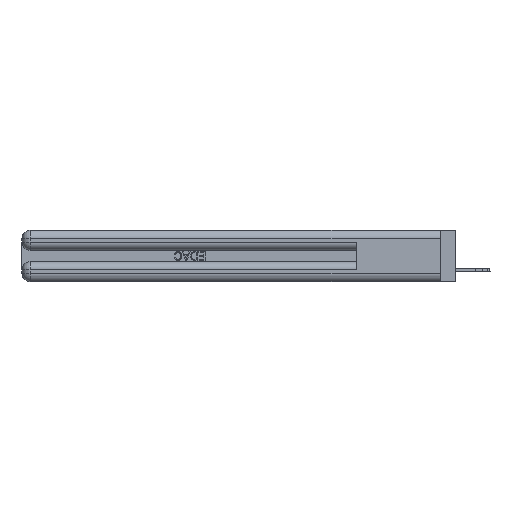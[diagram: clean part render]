
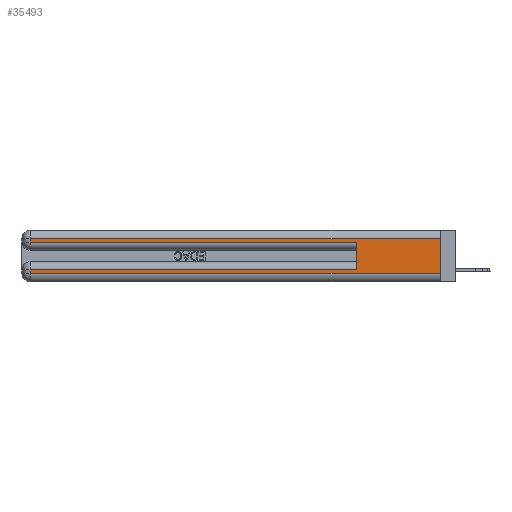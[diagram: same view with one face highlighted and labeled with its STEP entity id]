
A CAD part, left-side view. The second image highlights one B-rep face of the part: STEP entity #35493.
In plain terms, the highlighted planar face has unit normal (-1, 0, 0).
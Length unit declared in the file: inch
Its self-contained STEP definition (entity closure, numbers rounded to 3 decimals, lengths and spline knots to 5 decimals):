
#1325 = ORIENTED_EDGE ( 'NONE', *, *, #3280, .T. ) ;
#1948 = PLANE ( 'NONE',  #37656 ) ;
#2140 = DIRECTION ( 'NONE',  ( 0., 0., -1. ) ) ;
#2930 = VERTEX_POINT ( 'NONE', #23353 ) ;
#3280 = EDGE_CURVE ( 'NONE', #31481, #2930, #23337, .T. ) ;
#3364 = CARTESIAN_POINT ( 'NONE',  ( 0., 0., 0.31 ) ) ;
#3523 = VECTOR ( 'NONE', #14774, 39.37008 ) ;
#3614 = EDGE_CURVE ( 'NONE', #2930, #20798, #17515, .T. ) ;
#4989 = VECTOR ( 'NONE', #32613, 39.37008 ) ;
#5030 = CARTESIAN_POINT ( 'NONE',  ( 0., 0., 0.06 ) ) ;
#5789 = LINE ( 'NONE', #5030, #34237 ) ;
#6220 = LINE ( 'NONE', #10627, #21647 ) ;
#8026 = DIRECTION ( 'NONE',  ( 1., 0., 0. ) ) ;
#8174 = VECTOR ( 'NONE', #14922, 39.37008 ) ;
#8449 = ORIENTED_EDGE ( 'NONE', *, *, #36669, .T. ) ;
#8536 = VERTEX_POINT ( 'NONE', #16833 ) ;
#10357 = CARTESIAN_POINT ( 'NONE',  ( 0., 0., 0.31 ) ) ;
#10627 = CARTESIAN_POINT ( 'NONE',  ( 0., 0., 0.085 ) ) ;
#11812 = CARTESIAN_POINT ( 'NONE',  ( 0., 0.6, 0.145 ) ) ;
#11823 = CARTESIAN_POINT ( 'NONE',  ( 0., 2.94, 0.06 ) ) ;
#13100 = CARTESIAN_POINT ( 'NONE',  ( 0., 0., 0.37 ) ) ;
#13444 = VERTEX_POINT ( 'NONE', #30317 ) ;
#13823 = LINE ( 'NONE', #17106, #23493 ) ;
#13838 = VECTOR ( 'NONE', #22507, 39.37008 ) ;
#14729 = EDGE_CURVE ( 'NONE', #14881, #20798, #38062, .T. ) ;
#14774 = DIRECTION ( 'NONE',  ( 0., 0., -1. ) ) ;
#14881 = VERTEX_POINT ( 'NONE', #22222 ) ;
#14922 = DIRECTION ( 'NONE',  ( 0., 0., 1. ) ) ;
#14942 = ORIENTED_EDGE ( 'NONE', *, *, #26056, .T. ) ;
#15042 = EDGE_LOOP ( 'NONE', ( #24787, #33107, #1325, #31427, #30778, #14942, #8449, #38339 ) ) ;
#16712 = DIRECTION ( 'NONE',  ( 0., -1., 0. ) ) ;
#16833 = CARTESIAN_POINT ( 'NONE',  ( 0., 0., 0.06 ) ) ;
#17106 = CARTESIAN_POINT ( 'NONE',  ( 0., 2.94, 0.37 ) ) ;
#17515 = LINE ( 'NONE', #38099, #4989 ) ;
#18648 = VECTOR ( 'NONE', #34614, 39.37008 ) ;
#20024 = DIRECTION ( 'NONE',  ( 0., 0., -1. ) ) ;
#20262 = FACE_OUTER_BOUND ( 'NONE', #15042, .T. ) ;
#20798 = VERTEX_POINT ( 'NONE', #31462 ) ;
#21647 = VECTOR ( 'NONE', #35519, 39.37008 ) ;
#22222 = CARTESIAN_POINT ( 'NONE',  ( 0., 0.6, 0.085 ) ) ;
#22507 = DIRECTION ( 'NONE',  ( 0., 1., 0. ) ) ;
#23337 = LINE ( 'NONE', #33353, #3523 ) ;
#23353 = CARTESIAN_POINT ( 'NONE',  ( 0., 2.94, 0.285 ) ) ;
#23493 = VECTOR ( 'NONE', #2140, 39.37008 ) ;
#24787 = ORIENTED_EDGE ( 'NONE', *, *, #36968, .F. ) ;
#25267 = EDGE_CURVE ( 'NONE', #29333, #8536, #5789, .T. ) ;
#26056 = EDGE_CURVE ( 'NONE', #14881, #13444, #6220, .T. ) ;
#29333 = VERTEX_POINT ( 'NONE', #11823 ) ;
#30243 = EDGE_CURVE ( 'NONE', #30724, #31481, #36104, .T. ) ;
#30317 = CARTESIAN_POINT ( 'NONE',  ( 0., 2.94, 0.085 ) ) ;
#30724 = VERTEX_POINT ( 'NONE', #3364 ) ;
#30778 = ORIENTED_EDGE ( 'NONE', *, *, #14729, .F. ) ;
#31427 = ORIENTED_EDGE ( 'NONE', *, *, #3614, .T. ) ;
#31462 = CARTESIAN_POINT ( 'NONE',  ( 0., 0.6, 0.285 ) ) ;
#31481 = VERTEX_POINT ( 'NONE', #34067 ) ;
#32613 = DIRECTION ( 'NONE',  ( 0., -1., 0. ) ) ;
#33107 = ORIENTED_EDGE ( 'NONE', *, *, #30243, .T. ) ;
#33264 = LINE ( 'NONE', #13100, #18648 ) ;
#33353 = CARTESIAN_POINT ( 'NONE',  ( 0., 2.94, 0.37 ) ) ;
#34067 = CARTESIAN_POINT ( 'NONE',  ( 0., 2.94, 0.31 ) ) ;
#34237 = VECTOR ( 'NONE', #16712, 39.37008 ) ;
#34614 = DIRECTION ( 'NONE',  ( 0., 0., -1. ) ) ;
#35435 = CARTESIAN_POINT ( 'NONE',  ( 0., 0., 0.37 ) ) ;
#35493 = ADVANCED_FACE ( 'NONE', ( #20262 ), #1948, .F. ) ;
#35519 = DIRECTION ( 'NONE',  ( 0., 1., 0. ) ) ;
#36104 = LINE ( 'NONE', #10357, #13838 ) ;
#36669 = EDGE_CURVE ( 'NONE', #13444, #29333, #13823, .T. ) ;
#36968 = EDGE_CURVE ( 'NONE', #30724, #8536, #33264, .T. ) ;
#37656 = AXIS2_PLACEMENT_3D ( 'NONE', #35435, #8026, #20024 ) ;
#38062 = LINE ( 'NONE', #11812, #8174 ) ;
#38099 = CARTESIAN_POINT ( 'NONE',  ( 0., 0., 0.285 ) ) ;
#38339 = ORIENTED_EDGE ( 'NONE', *, *, #25267, .T. ) ;
